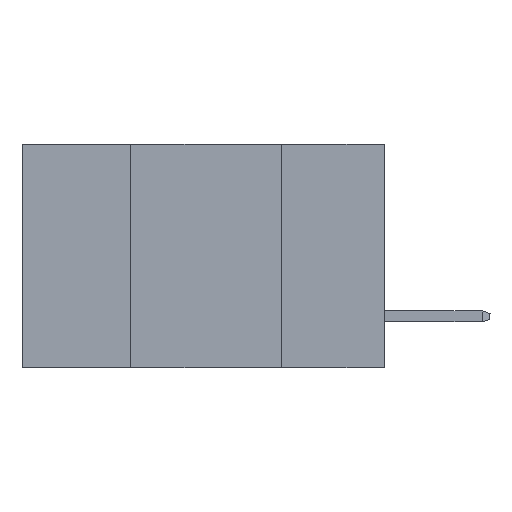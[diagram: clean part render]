
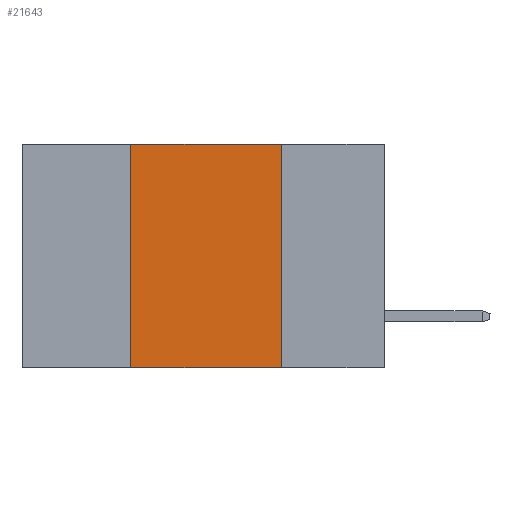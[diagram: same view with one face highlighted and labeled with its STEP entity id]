
A CAD part, left-side view. The second image highlights one B-rep face of the part: STEP entity #21643.
In plain terms, the highlighted planar face has unit normal (-1, 0, 0).
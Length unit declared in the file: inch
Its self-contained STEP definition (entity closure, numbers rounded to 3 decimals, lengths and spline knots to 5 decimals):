
#961 = VECTOR ( 'NONE', #19620, 39.37008 ) ;
#1194 = CARTESIAN_POINT ( 'NONE',  ( 0., 0.17, 0. ) ) ;
#1783 = DIRECTION ( 'NONE',  ( 0., 0., -1. ) ) ;
#2343 = LINE ( 'NONE', #13913, #7992 ) ;
#2977 = ORIENTED_EDGE ( 'NONE', *, *, #12576, .F. ) ;
#3472 = CARTESIAN_POINT ( 'NONE',  ( 0., 0.42, 0. ) ) ;
#4367 = LINE ( 'NONE', #15823, #24082 ) ;
#5677 = FACE_OUTER_BOUND ( 'NONE', #21108, .T. ) ;
#5688 = EDGE_CURVE ( 'NONE', #19172, #6005, #19753, .T. ) ;
#6005 = VERTEX_POINT ( 'NONE', #1194 ) ;
#6399 = ORIENTED_EDGE ( 'NONE', *, *, #22589, .T. ) ;
#7992 = VECTOR ( 'NONE', #14168, 39.37008 ) ;
#9776 = CARTESIAN_POINT ( 'NONE',  ( 0., 0.6, 0. ) ) ;
#9907 = DIRECTION ( 'NONE',  ( 0., 0., -1. ) ) ;
#10627 = VERTEX_POINT ( 'NONE', #15493 ) ;
#11565 = DIRECTION ( 'NONE',  ( 1., 0., 0. ) ) ;
#12012 = DIRECTION ( 'NONE',  ( 0., -1., 0. ) ) ;
#12038 = VECTOR ( 'NONE', #12012, 39.37008 ) ;
#12576 = EDGE_CURVE ( 'NONE', #6005, #10627, #4367, .T. ) ;
#13477 = PLANE ( 'NONE',  #14884 ) ;
#13563 = CARTESIAN_POINT ( 'NONE',  ( 0., 0.6, 0. ) ) ;
#13913 = CARTESIAN_POINT ( 'NONE',  ( 0., 0.42, -0.37 ) ) ;
#14168 = DIRECTION ( 'NONE',  ( 0., 0., 1. ) ) ;
#14884 = AXIS2_PLACEMENT_3D ( 'NONE', #9776, #11565, #1783 ) ;
#15493 = CARTESIAN_POINT ( 'NONE',  ( 0., 0.17, -0.37 ) ) ;
#15535 = CARTESIAN_POINT ( 'NONE',  ( 0., 0.42, -0.37 ) ) ;
#15823 = CARTESIAN_POINT ( 'NONE',  ( 0., 0.17, -0.37 ) ) ;
#16267 = LINE ( 'NONE', #23967, #12038 ) ;
#16694 = VERTEX_POINT ( 'NONE', #15535 ) ;
#19172 = VERTEX_POINT ( 'NONE', #3472 ) ;
#19620 = DIRECTION ( 'NONE',  ( 0., -1., 0. ) ) ;
#19753 = LINE ( 'NONE', #13563, #961 ) ;
#20379 = ORIENTED_EDGE ( 'NONE', *, *, #5688, .F. ) ;
#21108 = EDGE_LOOP ( 'NONE', ( #2977, #20379, #23988, #6399 ) ) ;
#21643 = ADVANCED_FACE ( 'NONE', ( #5677 ), #13477, .F. ) ;
#22589 = EDGE_CURVE ( 'NONE', #16694, #10627, #16267, .T. ) ;
#23077 = EDGE_CURVE ( 'NONE', #16694, #19172, #2343, .T. ) ;
#23967 = CARTESIAN_POINT ( 'NONE',  ( 0., 0.6, -0.37 ) ) ;
#23988 = ORIENTED_EDGE ( 'NONE', *, *, #23077, .F. ) ;
#24082 = VECTOR ( 'NONE', #9907, 39.37008 ) ;
